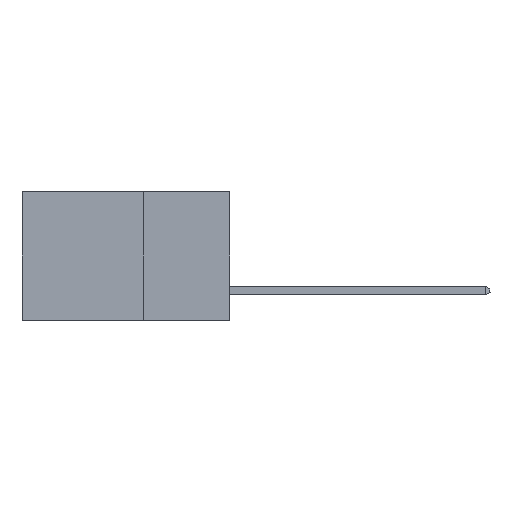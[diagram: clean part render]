
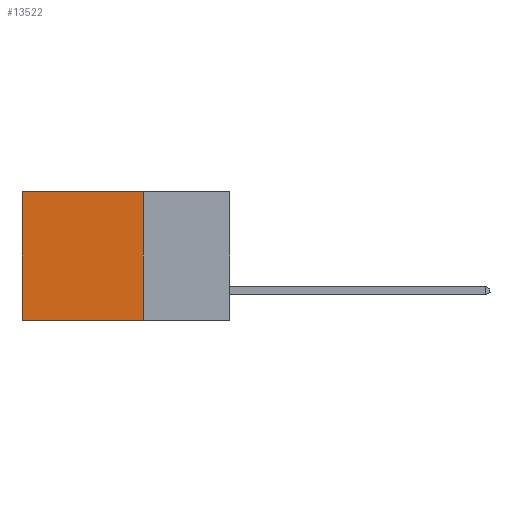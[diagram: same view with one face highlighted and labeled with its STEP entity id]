
A CAD part, left-side view. The second image highlights one B-rep face of the part: STEP entity #13522.
In plain terms, the highlighted planar face has unit normal (-1, 0, 0).
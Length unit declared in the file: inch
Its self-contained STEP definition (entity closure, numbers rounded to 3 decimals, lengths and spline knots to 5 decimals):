
#1673 = LINE ( 'NONE', #22187, #15624 ) ;
#1916 = VECTOR ( 'NONE', #8478, 39.37008 ) ;
#3845 = CARTESIAN_POINT ( 'NONE',  ( 0.298, 0.25, 0. ) ) ;
#5883 = AXIS2_PLACEMENT_3D ( 'NONE', #19173, #21291, #9526 ) ;
#6294 = DIRECTION ( 'NONE',  ( 0., 1., 0. ) ) ;
#8478 = DIRECTION ( 'NONE',  ( 0., 0., -1. ) ) ;
#9076 = CARTESIAN_POINT ( 'NONE',  ( 0.298, 0.25, 0. ) ) ;
#9526 = DIRECTION ( 'NONE',  ( 0., 0., -1. ) ) ;
#10831 = ORIENTED_EDGE ( 'NONE', *, *, #29873, .T. ) ;
#11208 = CARTESIAN_POINT ( 'NONE',  ( 0.298, 0.6, 0. ) ) ;
#11475 = CARTESIAN_POINT ( 'NONE',  ( 0.298, 0.25, 0. ) ) ;
#13522 = ADVANCED_FACE ( 'NONE', ( #30911 ), #18866, .F. ) ;
#13572 = VERTEX_POINT ( 'NONE', #17360 ) ;
#14402 = LINE ( 'NONE', #3845, #20833 ) ;
#15624 = VECTOR ( 'NONE', #29147, 39.37008 ) ;
#15910 = DIRECTION ( 'NONE',  ( 0., 0., -1. ) ) ;
#17195 = VERTEX_POINT ( 'NONE', #31223 ) ;
#17302 = VECTOR ( 'NONE', #15910, 39.37008 ) ;
#17360 = CARTESIAN_POINT ( 'NONE',  ( 0.298, 0.6, 0. ) ) ;
#17406 = ORIENTED_EDGE ( 'NONE', *, *, #30503, .T. ) ;
#17514 = VERTEX_POINT ( 'NONE', #20231 ) ;
#18075 = LINE ( 'NONE', #9076, #17302 ) ;
#18866 = PLANE ( 'NONE',  #5883 ) ;
#18874 = LINE ( 'NONE', #11208, #1916 ) ;
#19173 = CARTESIAN_POINT ( 'NONE',  ( 0.298, 0.25, 0. ) ) ;
#20231 = CARTESIAN_POINT ( 'NONE',  ( 0.298, 0.6, -0.37 ) ) ;
#20833 = VECTOR ( 'NONE', #6294, 39.37008 ) ;
#21291 = DIRECTION ( 'NONE',  ( 1., 0., 0. ) ) ;
#21355 = VERTEX_POINT ( 'NONE', #11475 ) ;
#22187 = CARTESIAN_POINT ( 'NONE',  ( 0.298, 0.25, -0.37 ) ) ;
#23154 = ORIENTED_EDGE ( 'NONE', *, *, #23615, .F. ) ;
#23615 = EDGE_CURVE ( 'NONE', #21355, #17195, #18075, .T. ) ;
#25603 = ORIENTED_EDGE ( 'NONE', *, *, #28538, .F. ) ;
#27269 = EDGE_LOOP ( 'NONE', ( #17406, #25603, #23154, #10831 ) ) ;
#28538 = EDGE_CURVE ( 'NONE', #17195, #17514, #1673, .T. ) ;
#29147 = DIRECTION ( 'NONE',  ( 0., 1., 0. ) ) ;
#29873 = EDGE_CURVE ( 'NONE', #21355, #13572, #14402, .T. ) ;
#30503 = EDGE_CURVE ( 'NONE', #13572, #17514, #18874, .T. ) ;
#30911 = FACE_OUTER_BOUND ( 'NONE', #27269, .T. ) ;
#31223 = CARTESIAN_POINT ( 'NONE',  ( 0.298, 0.25, -0.37 ) ) ;
